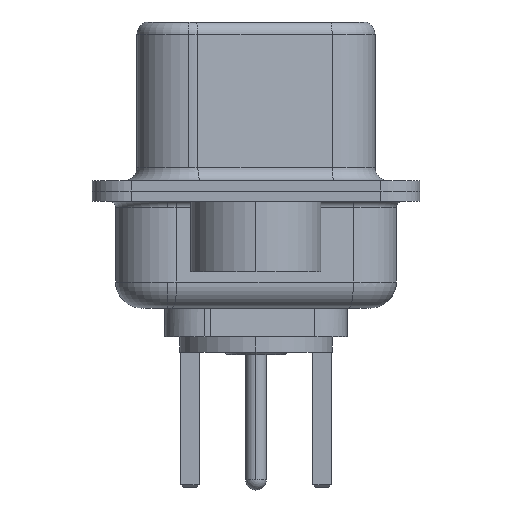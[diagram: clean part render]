
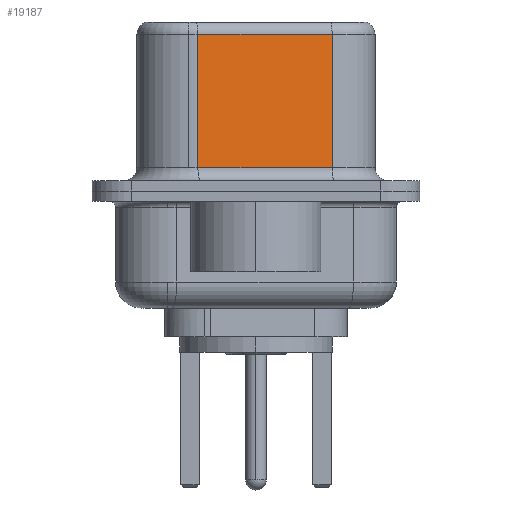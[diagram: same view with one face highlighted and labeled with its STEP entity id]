
A CAD part, left-side view. The second image highlights one B-rep face of the part: STEP entity #19187.
In plain terms, the highlighted planar face has unit normal (-0.985, -0.174, 0).
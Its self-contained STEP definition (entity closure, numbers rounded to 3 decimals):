
#595 = FACE_OUTER_BOUND ( 'NONE', #16852, .T. ) ;
#1114 = CARTESIAN_POINT ( 'NONE',  ( 4.58, -2.927, 6.52 ) ) ;
#1377 = CARTESIAN_POINT ( 'NONE',  ( 4.58, -2.927, 6.02 ) ) ;
#1722 = VERTEX_POINT ( 'NONE', #15381 ) ;
#2715 = CARTESIAN_POINT ( 'NONE',  ( 3.67, 2.233, 0.9 ) ) ;
#2971 = VECTOR ( 'NONE', #10912, 1000. ) ;
#4313 = EDGE_CURVE ( 'NONE', #10131, #1722, #13292, .T. ) ;
#4546 = ORIENTED_EDGE ( 'NONE', *, *, #11952, .F. ) ;
#4739 = ORIENTED_EDGE ( 'NONE', *, *, #10791, .T. ) ;
#5207 = ORIENTED_EDGE ( 'NONE', *, *, #13001, .T. ) ;
#5332 = ORIENTED_EDGE ( 'NONE', *, *, #4313, .T. ) ;
#7832 = LINE ( 'NONE', #1114, #2971 ) ;
#8089 = VECTOR ( 'NONE', #20936, 1000. ) ;
#8098 = VERTEX_POINT ( 'NONE', #9667 ) ;
#8461 = DIRECTION ( 'NONE',  ( 0.985, 0.174, 0. ) ) ;
#8637 = CARTESIAN_POINT ( 'NONE',  ( 4.58, -2.927, 6.02 ) ) ;
#9593 = DIRECTION ( 'NONE',  ( -0.174, 0.985, 0. ) ) ;
#9667 = CARTESIAN_POINT ( 'NONE',  ( 3.67, 2.233, 6.02 ) ) ;
#10131 = VERTEX_POINT ( 'NONE', #2715 ) ;
#10791 = EDGE_CURVE ( 'NONE', #14971, #8098, #12949, .T. ) ;
#10912 = DIRECTION ( 'NONE',  ( 0., 0., -1. ) ) ;
#11406 = CARTESIAN_POINT ( 'NONE',  ( 3.67, 2.233, 6.52 ) ) ;
#11952 = EDGE_CURVE ( 'NONE', #14971, #1722, #7832, .T. ) ;
#12761 = VECTOR ( 'NONE', #18242, 1000. ) ;
#12949 = LINE ( 'NONE', #1377, #16657 ) ;
#13001 = EDGE_CURVE ( 'NONE', #8098, #10131, #19874, .T. ) ;
#13292 = LINE ( 'NONE', #15199, #12761 ) ;
#14895 = PLANE ( 'NONE',  #19095 ) ;
#14971 = VERTEX_POINT ( 'NONE', #8637 ) ;
#15199 = CARTESIAN_POINT ( 'NONE',  ( 4.58, -2.927, 0.9 ) ) ;
#15381 = CARTESIAN_POINT ( 'NONE',  ( 4.58, -2.927, 0.9 ) ) ;
#16657 = VECTOR ( 'NONE', #9593, 1000. ) ;
#16852 = EDGE_LOOP ( 'NONE', ( #4546, #4739, #5207, #5332 ) ) ;
#18074 = CARTESIAN_POINT ( 'NONE',  ( 4.58, -2.927, 6.52 ) ) ;
#18242 = DIRECTION ( 'NONE',  ( 0.174, -0.985, 0. ) ) ;
#19095 = AXIS2_PLACEMENT_3D ( 'NONE', #18074, #8461, #19677 ) ;
#19187 = ADVANCED_FACE ( 'NONE', ( #595 ), #14895, .F. ) ;
#19677 = DIRECTION ( 'NONE',  ( -0.174, 0.985, 0. ) ) ;
#19874 = LINE ( 'NONE', #11406, #8089 ) ;
#20936 = DIRECTION ( 'NONE',  ( 0., 0., -1. ) ) ;
